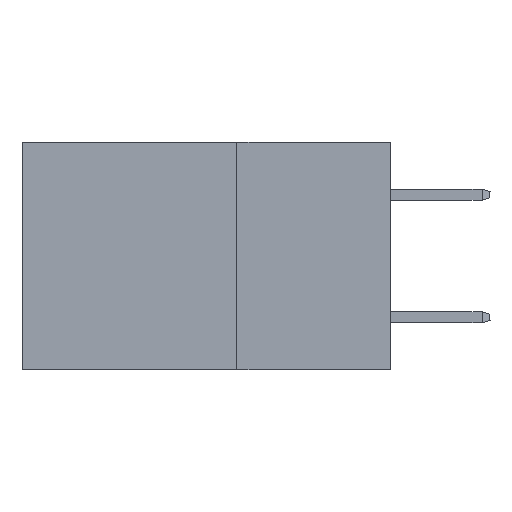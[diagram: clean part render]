
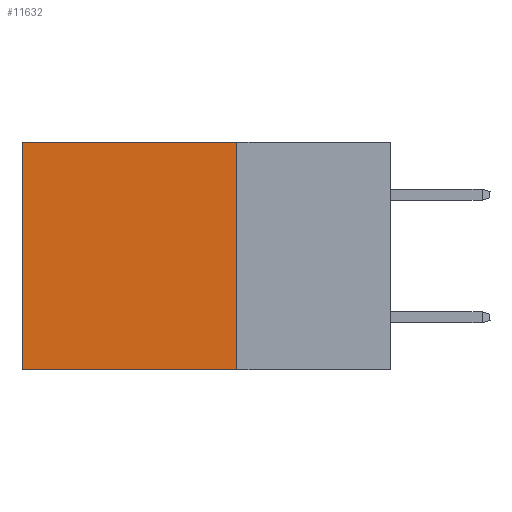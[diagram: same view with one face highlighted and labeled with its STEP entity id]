
A CAD part, left-side view. The second image highlights one B-rep face of the part: STEP entity #11632.
In plain terms, the highlighted planar face has unit normal (-1, 0, 0).
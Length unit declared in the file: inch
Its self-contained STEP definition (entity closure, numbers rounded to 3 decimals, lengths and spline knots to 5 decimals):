
#689 = DIRECTION ( 'NONE',  ( 0., 0., -1. ) ) ;
#817 = VERTEX_POINT ( 'NONE', #6797 ) ;
#907 = EDGE_CURVE ( 'NONE', #13994, #7864, #18338, .T. ) ;
#944 = DIRECTION ( 'NONE',  ( 0., 0., -1. ) ) ;
#1372 = EDGE_LOOP ( 'NONE', ( #7193, #14952, #3572, #10292 ) ) ;
#2713 = CARTESIAN_POINT ( 'NONE',  ( 0.2875, 0.6, 0. ) ) ;
#2854 = DIRECTION ( 'NONE',  ( 0., 0., -1. ) ) ;
#3400 = LINE ( 'NONE', #6390, #17042 ) ;
#3572 = ORIENTED_EDGE ( 'NONE', *, *, #12406, .F. ) ;
#3637 = FACE_OUTER_BOUND ( 'NONE', #1372, .T. ) ;
#3727 = DIRECTION ( 'NONE',  ( 1., 0., 0. ) ) ;
#4396 = VECTOR ( 'NONE', #17346, 39.37008 ) ;
#6390 = CARTESIAN_POINT ( 'NONE',  ( 0.2875, 0.25, 0. ) ) ;
#6616 = DIRECTION ( 'NONE',  ( 0., 1., 0. ) ) ;
#6797 = CARTESIAN_POINT ( 'NONE',  ( 0.2875, 0.25, 0. ) ) ;
#7130 = EDGE_CURVE ( 'NONE', #817, #13994, #8263, .T. ) ;
#7193 = ORIENTED_EDGE ( 'NONE', *, *, #907, .T. ) ;
#7864 = VERTEX_POINT ( 'NONE', #12197 ) ;
#8072 = CARTESIAN_POINT ( 'NONE',  ( 0.2875, 0.25, -0.37 ) ) ;
#8263 = LINE ( 'NONE', #14175, #9812 ) ;
#9812 = VECTOR ( 'NONE', #6616, 39.37008 ) ;
#10080 = VECTOR ( 'NONE', #689, 39.37008 ) ;
#10292 = ORIENTED_EDGE ( 'NONE', *, *, #7130, .T. ) ;
#10991 = CARTESIAN_POINT ( 'NONE',  ( 0.2875, 0.6, 0. ) ) ;
#11111 = CARTESIAN_POINT ( 'NONE',  ( 0.2875, 0.25, 0. ) ) ;
#11632 = ADVANCED_FACE ( 'NONE', ( #3637 ), #12360, .F. ) ;
#12197 = CARTESIAN_POINT ( 'NONE',  ( 0.2875, 0.6, -0.37 ) ) ;
#12360 = PLANE ( 'NONE',  #14226 ) ;
#12406 = EDGE_CURVE ( 'NONE', #817, #13389, #3400, .T. ) ;
#13094 = LINE ( 'NONE', #16089, #4396 ) ;
#13389 = VERTEX_POINT ( 'NONE', #8072 ) ;
#13994 = VERTEX_POINT ( 'NONE', #2713 ) ;
#14175 = CARTESIAN_POINT ( 'NONE',  ( 0.2875, 0.25, 0. ) ) ;
#14226 = AXIS2_PLACEMENT_3D ( 'NONE', #11111, #3727, #2854 ) ;
#14952 = ORIENTED_EDGE ( 'NONE', *, *, #16732, .F. ) ;
#16089 = CARTESIAN_POINT ( 'NONE',  ( 0.2875, 0.25, -0.37 ) ) ;
#16732 = EDGE_CURVE ( 'NONE', #13389, #7864, #13094, .T. ) ;
#17042 = VECTOR ( 'NONE', #944, 39.37008 ) ;
#17346 = DIRECTION ( 'NONE',  ( 0., 1., 0. ) ) ;
#18338 = LINE ( 'NONE', #10991, #10080 ) ;
